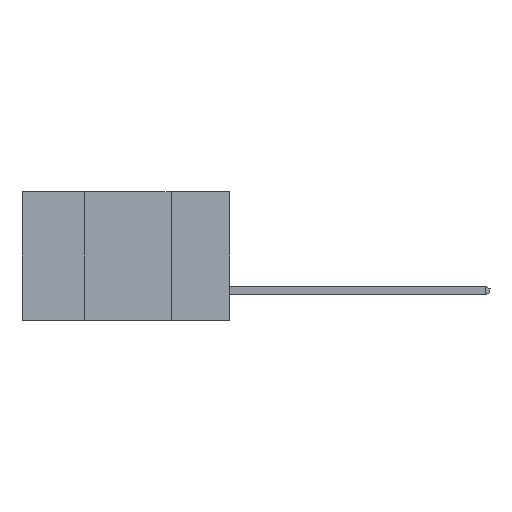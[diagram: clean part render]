
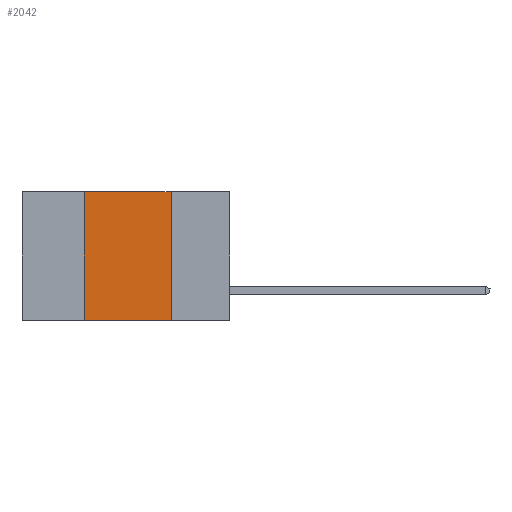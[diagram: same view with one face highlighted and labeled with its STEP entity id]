
A CAD part, left-side view. The second image highlights one B-rep face of the part: STEP entity #2042.
In plain terms, the highlighted planar face has unit normal (-1, 0, 0).
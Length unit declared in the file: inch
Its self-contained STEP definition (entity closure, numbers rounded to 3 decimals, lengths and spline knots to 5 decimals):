
#52 = AXIS2_PLACEMENT_3D ( 'NONE', #7802, #6911, #10526 ) ;
#422 = LINE ( 'NONE', #3965, #874 ) ;
#874 = VECTOR ( 'NONE', #3064, 39.37008 ) ;
#1062 = VERTEX_POINT ( 'NONE', #2201 ) ;
#1445 = LINE ( 'NONE', #6591, #3258 ) ;
#1468 = ORIENTED_EDGE ( 'NONE', *, *, #10798, .F. ) ;
#1846 = VERTEX_POINT ( 'NONE', #10375 ) ;
#2042 = ADVANCED_FACE ( 'NONE', ( #7852 ), #4230, .F. ) ;
#2201 = CARTESIAN_POINT ( 'NONE',  ( 0., 0.42, -0.37 ) ) ;
#2309 = EDGE_CURVE ( 'NONE', #1062, #4678, #7601, .T. ) ;
#2364 = VECTOR ( 'NONE', #8225, 39.37008 ) ;
#3064 = DIRECTION ( 'NONE',  ( 0., 0., -1. ) ) ;
#3258 = VECTOR ( 'NONE', #6640, 39.37008 ) ;
#3360 = CARTESIAN_POINT ( 'NONE',  ( 0., 0.42, 0. ) ) ;
#3965 = CARTESIAN_POINT ( 'NONE',  ( 0., 0.17, -0.37 ) ) ;
#4230 = PLANE ( 'NONE',  #52 ) ;
#4678 = VERTEX_POINT ( 'NONE', #8078 ) ;
#5391 = LINE ( 'NONE', #6337, #2364 ) ;
#5651 = VECTOR ( 'NONE', #7543, 39.37008 ) ;
#6337 = CARTESIAN_POINT ( 'NONE',  ( 0., 0.6, 0. ) ) ;
#6591 = CARTESIAN_POINT ( 'NONE',  ( 0., 0.42, -0.37 ) ) ;
#6640 = DIRECTION ( 'NONE',  ( 0., 0., 1. ) ) ;
#6911 = DIRECTION ( 'NONE',  ( 1., 0., 0. ) ) ;
#7543 = DIRECTION ( 'NONE',  ( 0., -1., 0. ) ) ;
#7601 = LINE ( 'NONE', #8608, #5651 ) ;
#7785 = ORIENTED_EDGE ( 'NONE', *, *, #11329, .F. ) ;
#7802 = CARTESIAN_POINT ( 'NONE',  ( 0., 0.6, 0. ) ) ;
#7852 = FACE_OUTER_BOUND ( 'NONE', #9546, .T. ) ;
#8078 = CARTESIAN_POINT ( 'NONE',  ( 0., 0.17, -0.37 ) ) ;
#8225 = DIRECTION ( 'NONE',  ( 0., -1., 0. ) ) ;
#8608 = CARTESIAN_POINT ( 'NONE',  ( 0., 0.6, -0.37 ) ) ;
#8714 = ORIENTED_EDGE ( 'NONE', *, *, #8801, .F. ) ;
#8801 = EDGE_CURVE ( 'NONE', #1062, #10018, #1445, .T. ) ;
#9406 = ORIENTED_EDGE ( 'NONE', *, *, #2309, .T. ) ;
#9546 = EDGE_LOOP ( 'NONE', ( #1468, #7785, #8714, #9406 ) ) ;
#10018 = VERTEX_POINT ( 'NONE', #3360 ) ;
#10375 = CARTESIAN_POINT ( 'NONE',  ( 0., 0.17, 0. ) ) ;
#10526 = DIRECTION ( 'NONE',  ( 0., 0., -1. ) ) ;
#10798 = EDGE_CURVE ( 'NONE', #1846, #4678, #422, .T. ) ;
#11329 = EDGE_CURVE ( 'NONE', #10018, #1846, #5391, .T. ) ;
